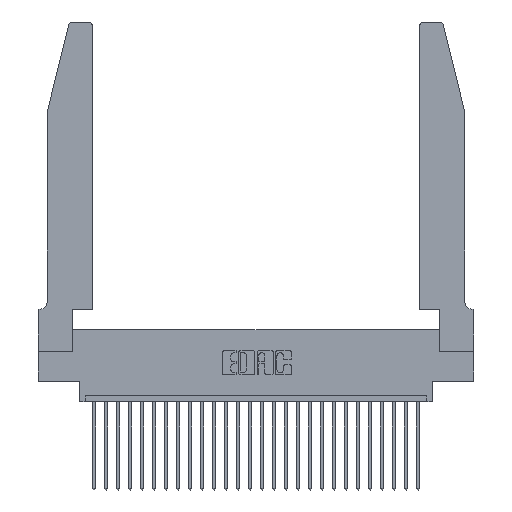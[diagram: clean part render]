
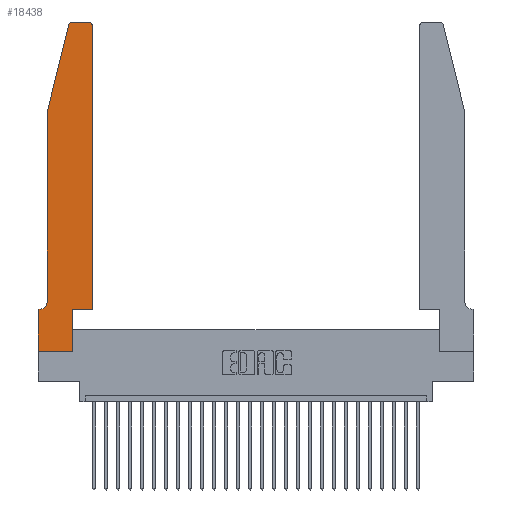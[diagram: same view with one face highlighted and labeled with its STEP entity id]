
A CAD part, top view. The second image highlights one B-rep face of the part: STEP entity #18438.
In plain terms, the highlighted planar face has unit normal (0, 0, 1).
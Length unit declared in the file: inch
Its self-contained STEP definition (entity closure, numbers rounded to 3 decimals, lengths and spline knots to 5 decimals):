
#585 = VECTOR ( 'NONE', #14350, 39.37008 ) ;
#594 = CARTESIAN_POINT ( 'NONE',  ( 0.2865, 0.35, 0.37 ) ) ;
#965 = ORIENTED_EDGE ( 'NONE', *, *, #16091, .T. ) ;
#1387 = VERTEX_POINT ( 'NONE', #16190 ) ;
#1413 = CARTESIAN_POINT ( 'NONE',  ( 0.0755, 0.35, 0.37 ) ) ;
#1470 = CARTESIAN_POINT ( 'NONE',  ( 0.4505, 0.35, 0.37 ) ) ;
#1628 = CARTESIAN_POINT ( 'NONE',  ( 0.2605, 2.75, 0.37 ) ) ;
#1745 = EDGE_CURVE ( 'NONE', #1387, #15200, #3624, .T. ) ;
#2047 = DIRECTION ( 'NONE',  ( 1., 0., 0. ) ) ;
#2434 = DIRECTION ( 'NONE',  ( 0., -1., 0. ) ) ;
#3284 = VECTOR ( 'NONE', #14567, 39.37008 ) ;
#3413 = CARTESIAN_POINT ( 'NONE',  ( 0., 0.35, 0.37 ) ) ;
#3624 = LINE ( 'NONE', #1628, #585 ) ;
#3839 = VECTOR ( 'NONE', #5690, 39.37008 ) ;
#4323 = EDGE_CURVE ( 'NONE', #22814, #26599, #21694, .T. ) ;
#4565 = VERTEX_POINT ( 'NONE', #21650 ) ;
#5651 = EDGE_CURVE ( 'NONE', #27106, #4565, #15941, .T. ) ;
#5690 = DIRECTION ( 'NONE',  ( -1., 0., 0. ) ) ;
#6654 = DIRECTION ( 'NONE',  ( 0., 0., -1. ) ) ;
#7062 = ORIENTED_EDGE ( 'NONE', *, *, #13778, .T. ) ;
#7325 = DIRECTION ( 'NONE',  ( -0.239, -0.971, 0. ) ) ;
#7612 = LINE ( 'NONE', #8722, #8306 ) ;
#7752 = ORIENTED_EDGE ( 'NONE', *, *, #20084, .T. ) ;
#7865 = EDGE_CURVE ( 'NONE', #16613, #14557, #27596, .T. ) ;
#7931 = DIRECTION ( 'NONE',  ( 1., 0., 0. ) ) ;
#8306 = VECTOR ( 'NONE', #15114, 39.37008 ) ;
#8722 = CARTESIAN_POINT ( 'NONE',  ( 0., 0., 0.37 ) ) ;
#8918 = LINE ( 'NONE', #17171, #10958 ) ;
#8970 = CARTESIAN_POINT ( 'NONE',  ( 0.2865, 0., 0.37 ) ) ;
#9106 = CIRCLE ( 'NONE', #21151, 0.07 ) ;
#9935 = AXIS2_PLACEMENT_3D ( 'NONE', #12184, #14322, #7931 ) ;
#10035 = DIRECTION ( 'NONE',  ( 0., 0., 1. ) ) ;
#10427 = CARTESIAN_POINT ( 'NONE',  ( 0., 0., 0.37 ) ) ;
#10534 = AXIS2_PLACEMENT_3D ( 'NONE', #10652, #25637, #2047 ) ;
#10652 = CARTESIAN_POINT ( 'NONE',  ( 0.4205, 2.72, 0.37 ) ) ;
#10958 = VECTOR ( 'NONE', #23995, 39.37008 ) ;
#11093 = CARTESIAN_POINT ( 'NONE',  ( 0.4505, 2.72, 0.37 ) ) ;
#12158 = CARTESIAN_POINT ( 'NONE',  ( 0.0755, 0.42, 0.37 ) ) ;
#12184 = CARTESIAN_POINT ( 'NONE',  ( 0.284, 2.72, 0.37 ) ) ;
#12634 = CIRCLE ( 'NONE', #10534, 0.03 ) ;
#13100 = ORIENTED_EDGE ( 'NONE', *, *, #24426, .T. ) ;
#13115 = ORIENTED_EDGE ( 'NONE', *, *, #5651, .T. ) ;
#13486 = CARTESIAN_POINT ( 'NONE',  ( 0.25487, 2.72718, 0.37 ) ) ;
#13609 = CARTESIAN_POINT ( 'NONE',  ( 0., 0.35, 0.37 ) ) ;
#13778 = EDGE_CURVE ( 'NONE', #14557, #1387, #12634, .T. ) ;
#13786 = CARTESIAN_POINT ( 'NONE',  ( 0.2865, 0.35, 0.37 ) ) ;
#13984 = CARTESIAN_POINT ( 'NONE',  ( 0.284, 2.75, 0.37 ) ) ;
#14047 = CARTESIAN_POINT ( 'NONE',  ( 0.0055, 0.35, 0.37 ) ) ;
#14322 = DIRECTION ( 'NONE',  ( 0., 0., 1. ) ) ;
#14350 = DIRECTION ( 'NONE',  ( -1., 0., 0. ) ) ;
#14557 = VERTEX_POINT ( 'NONE', #11093 ) ;
#14567 = DIRECTION ( 'NONE',  ( 1., 0., 0. ) ) ;
#15114 = DIRECTION ( 'NONE',  ( 1., 0., 0. ) ) ;
#15200 = VERTEX_POINT ( 'NONE', #13984 ) ;
#15237 = ORIENTED_EDGE ( 'NONE', *, *, #4323, .T. ) ;
#15844 = CARTESIAN_POINT ( 'NONE',  ( 0.4505, 0.35, 0.37 ) ) ;
#15941 = LINE ( 'NONE', #20189, #21657 ) ;
#16091 = EDGE_CURVE ( 'NONE', #16797, #22814, #9106, .T. ) ;
#16181 = VECTOR ( 'NONE', #22994, 39.37008 ) ;
#16190 = CARTESIAN_POINT ( 'NONE',  ( 0.4205, 2.75, 0.37 ) ) ;
#16282 = EDGE_CURVE ( 'NONE', #27713, #26610, #18465, .T. ) ;
#16590 = PLANE ( 'NONE',  #24575 ) ;
#16613 = VERTEX_POINT ( 'NONE', #15844 ) ;
#16797 = VERTEX_POINT ( 'NONE', #12158 ) ;
#17171 = CARTESIAN_POINT ( 'NONE',  ( 0., 0., 0.37 ) ) ;
#17503 = VECTOR ( 'NONE', #26228, 39.37008 ) ;
#18438 = ADVANCED_FACE ( 'NONE', ( #22953 ), #16590, .T. ) ;
#18465 = LINE ( 'NONE', #594, #17503 ) ;
#19333 = LINE ( 'NONE', #25928, #24033 ) ;
#20036 = CIRCLE ( 'NONE', #9935, 0.03 ) ;
#20039 = ORIENTED_EDGE ( 'NONE', *, *, #26486, .T. ) ;
#20084 = EDGE_CURVE ( 'NONE', #26599, #25197, #8918, .T. ) ;
#20189 = CARTESIAN_POINT ( 'NONE',  ( 0.0755, 2., 0.37 ) ) ;
#20433 = DIRECTION ( 'NONE',  ( 1., 0., 0. ) ) ;
#21145 = ORIENTED_EDGE ( 'NONE', *, *, #7865, .T. ) ;
#21151 = AXIS2_PLACEMENT_3D ( 'NONE', #25696, #6654, #25880 ) ;
#21650 = CARTESIAN_POINT ( 'NONE',  ( 0.0755, 2., 0.37 ) ) ;
#21657 = VECTOR ( 'NONE', #7325, 39.37008 ) ;
#21694 = LINE ( 'NONE', #1413, #3839 ) ;
#22517 = EDGE_CURVE ( 'NONE', #25197, #27713, #7612, .T. ) ;
#22745 = EDGE_CURVE ( 'NONE', #15200, #27106, #20036, .T. ) ;
#22814 = VERTEX_POINT ( 'NONE', #14047 ) ;
#22901 = CARTESIAN_POINT ( 'NONE',  ( 0.4505, 0.35, 0.37 ) ) ;
#22953 = FACE_OUTER_BOUND ( 'NONE', #27754, .T. ) ;
#22994 = DIRECTION ( 'NONE',  ( 0., 1., 0. ) ) ;
#23220 = ORIENTED_EDGE ( 'NONE', *, *, #22745, .T. ) ;
#23482 = LINE ( 'NONE', #1470, #3284 ) ;
#23912 = ORIENTED_EDGE ( 'NONE', *, *, #22517, .T. ) ;
#23995 = DIRECTION ( 'NONE',  ( 0., -1., 0. ) ) ;
#24033 = VECTOR ( 'NONE', #2434, 39.37008 ) ;
#24426 = EDGE_CURVE ( 'NONE', #26610, #16613, #23482, .T. ) ;
#24575 = AXIS2_PLACEMENT_3D ( 'NONE', #3413, #10035, #20433 ) ;
#24607 = ORIENTED_EDGE ( 'NONE', *, *, #16282, .T. ) ;
#25197 = VERTEX_POINT ( 'NONE', #10427 ) ;
#25596 = ORIENTED_EDGE ( 'NONE', *, *, #1745, .T. ) ;
#25637 = DIRECTION ( 'NONE',  ( 0., 0., 1. ) ) ;
#25696 = CARTESIAN_POINT ( 'NONE',  ( 0.0055, 0.42, 0.37 ) ) ;
#25880 = DIRECTION ( 'NONE',  ( -1., 0., 0. ) ) ;
#25928 = CARTESIAN_POINT ( 'NONE',  ( 0.0755, 2., 0.37 ) ) ;
#26228 = DIRECTION ( 'NONE',  ( 0., 1., 0. ) ) ;
#26486 = EDGE_CURVE ( 'NONE', #4565, #16797, #19333, .T. ) ;
#26599 = VERTEX_POINT ( 'NONE', #13609 ) ;
#26610 = VERTEX_POINT ( 'NONE', #13786 ) ;
#27106 = VERTEX_POINT ( 'NONE', #13486 ) ;
#27596 = LINE ( 'NONE', #22901, #16181 ) ;
#27713 = VERTEX_POINT ( 'NONE', #8970 ) ;
#27754 = EDGE_LOOP ( 'NONE', ( #25596, #23220, #13115, #20039, #965, #15237, #7752, #23912, #24607, #13100, #21145, #7062 ) ) ;
